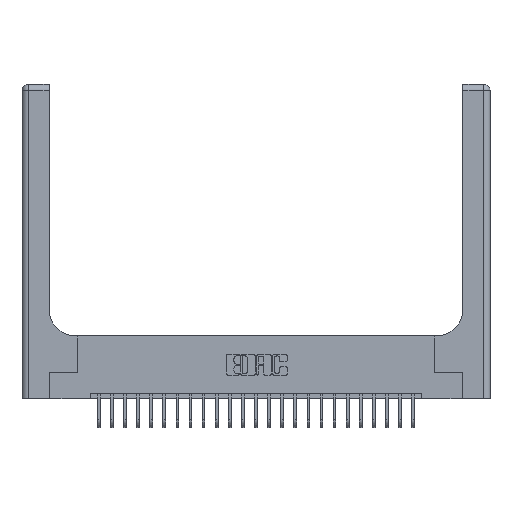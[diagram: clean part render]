
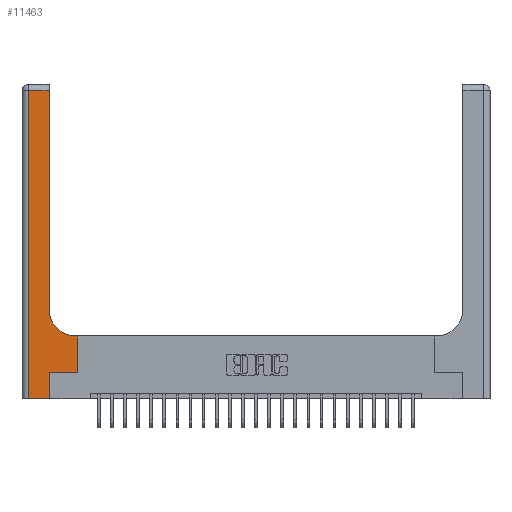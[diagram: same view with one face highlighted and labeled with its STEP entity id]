
A CAD part, top view. The second image highlights one B-rep face of the part: STEP entity #11463.
In plain terms, the highlighted planar face has unit normal (0, 0, 1).
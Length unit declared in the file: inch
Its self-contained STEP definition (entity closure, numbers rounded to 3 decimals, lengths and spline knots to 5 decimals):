
#179 = DIRECTION ( 'NONE',  ( 1., 0., 0. ) ) ;
#959 = CARTESIAN_POINT ( 'NONE',  ( 0.265, 0., 0.37 ) ) ;
#1138 = VERTEX_POINT ( 'NONE', #7204 ) ;
#1394 = LINE ( 'NONE', #23034, #22798 ) ;
#1745 = VERTEX_POINT ( 'NONE', #2069 ) ;
#1804 = ORIENTED_EDGE ( 'NONE', *, *, #21314, .T. ) ;
#2069 = CARTESIAN_POINT ( 'NONE',  ( 0.26, 2.94, 0.37 ) ) ;
#2202 = VERTEX_POINT ( 'NONE', #959 ) ;
#2420 = VECTOR ( 'NONE', #19166, 39.37008 ) ;
#2476 = DIRECTION ( 'NONE',  ( 0., 0., -1. ) ) ;
#2737 = VECTOR ( 'NONE', #9214, 39.37008 ) ;
#3122 = CIRCLE ( 'NONE', #4648, 0.25 ) ;
#3343 = AXIS2_PLACEMENT_3D ( 'NONE', #16476, #2476, #16950 ) ;
#3345 = ORIENTED_EDGE ( 'NONE', *, *, #22056, .T. ) ;
#3838 = CARTESIAN_POINT ( 'NONE',  ( 0.265, 0.25, 0.37 ) ) ;
#4006 = LINE ( 'NONE', #11257, #11906 ) ;
#4091 = LINE ( 'NONE', #20139, #2737 ) ;
#4648 = AXIS2_PLACEMENT_3D ( 'NONE', #20029, #17766, #179 ) ;
#4684 = CARTESIAN_POINT ( 'NONE',  ( 0.265, 0., 0.37 ) ) ;
#4686 = VECTOR ( 'NONE', #21534, 39.37008 ) ;
#5141 = ORIENTED_EDGE ( 'NONE', *, *, #15487, .T. ) ;
#5662 = ORIENTED_EDGE ( 'NONE', *, *, #13531, .T. ) ;
#5741 = CARTESIAN_POINT ( 'NONE',  ( 0.26, 0.6, 0.37 ) ) ;
#7204 = CARTESIAN_POINT ( 'NONE',  ( 0.26, 0.85, 0.37 ) ) ;
#7446 = ORIENTED_EDGE ( 'NONE', *, *, #13442, .T. ) ;
#8246 = VECTOR ( 'NONE', #8964, 39.37008 ) ;
#8887 = DIRECTION ( 'NONE',  ( 0., 1., 0. ) ) ;
#8964 = DIRECTION ( 'NONE',  ( -1., 0., 0. ) ) ;
#8998 = DIRECTION ( 'NONE',  ( -1., 0., 0. ) ) ;
#9214 = DIRECTION ( 'NONE',  ( 0., -1., 0. ) ) ;
#9449 = VECTOR ( 'NONE', #9553, 39.37008 ) ;
#9553 = DIRECTION ( 'NONE',  ( 1., 0., 0. ) ) ;
#9569 = EDGE_CURVE ( 'NONE', #12038, #19665, #18457, .T. ) ;
#9696 = CARTESIAN_POINT ( 'NONE',  ( 0.528, 0.25, 0.37 ) ) ;
#10384 = DIRECTION ( 'NONE',  ( 1., 0., 0. ) ) ;
#10613 = LINE ( 'NONE', #19649, #17385 ) ;
#10897 = ORIENTED_EDGE ( 'NONE', *, *, #22872, .T. ) ;
#11257 = CARTESIAN_POINT ( 'NONE',  ( 0.528, 0.25, 0.37 ) ) ;
#11463 = ADVANCED_FACE ( 'NONE', ( #18506 ), #18740, .F. ) ;
#11906 = VECTOR ( 'NONE', #8887, 39.37008 ) ;
#12038 = VERTEX_POINT ( 'NONE', #18829 ) ;
#12727 = CARTESIAN_POINT ( 'NONE',  ( 0.26, 3., 0.37 ) ) ;
#12927 = EDGE_LOOP ( 'NONE', ( #3345, #5141, #17344, #7446, #20315, #5662, #10897, #23105, #1804 ) ) ;
#13080 = VERTEX_POINT ( 'NONE', #18246 ) ;
#13442 = EDGE_CURVE ( 'NONE', #19148, #2202, #10613, .T. ) ;
#13531 = EDGE_CURVE ( 'NONE', #16179, #17462, #14645, .T. ) ;
#14645 = LINE ( 'NONE', #3838, #9449 ) ;
#15487 = EDGE_CURVE ( 'NONE', #1745, #13080, #1394, .T. ) ;
#15999 = CARTESIAN_POINT ( 'NONE',  ( 0.51, 0.6, 0.37 ) ) ;
#16179 = VERTEX_POINT ( 'NONE', #19897 ) ;
#16476 = CARTESIAN_POINT ( 'NONE',  ( 0., 3., 0.37 ) ) ;
#16950 = DIRECTION ( 'NONE',  ( -1., 0., 0. ) ) ;
#17121 = CARTESIAN_POINT ( 'NONE',  ( 0.06, 0., 0.37 ) ) ;
#17344 = ORIENTED_EDGE ( 'NONE', *, *, #17358, .T. ) ;
#17358 = EDGE_CURVE ( 'NONE', #13080, #19148, #4091, .T. ) ;
#17385 = VECTOR ( 'NONE', #10384, 39.37008 ) ;
#17462 = VERTEX_POINT ( 'NONE', #9696 ) ;
#17766 = DIRECTION ( 'NONE',  ( 0., 0., -1. ) ) ;
#18246 = CARTESIAN_POINT ( 'NONE',  ( 0.06, 2.94, 0.37 ) ) ;
#18457 = LINE ( 'NONE', #5741, #8246 ) ;
#18506 = FACE_OUTER_BOUND ( 'NONE', #12927, .T. ) ;
#18740 = PLANE ( 'NONE',  #3343 ) ;
#18829 = CARTESIAN_POINT ( 'NONE',  ( 0.528, 0.6, 0.37 ) ) ;
#18868 = EDGE_CURVE ( 'NONE', #2202, #16179, #20958, .T. ) ;
#19148 = VERTEX_POINT ( 'NONE', #17121 ) ;
#19166 = DIRECTION ( 'NONE',  ( 0., 1., 0. ) ) ;
#19649 = CARTESIAN_POINT ( 'NONE',  ( 0., 0., 0.37 ) ) ;
#19665 = VERTEX_POINT ( 'NONE', #15999 ) ;
#19897 = CARTESIAN_POINT ( 'NONE',  ( 0.265, 0.25, 0.37 ) ) ;
#20029 = CARTESIAN_POINT ( 'NONE',  ( 0.51, 0.85, 0.37 ) ) ;
#20139 = CARTESIAN_POINT ( 'NONE',  ( 0.06, 3., 0.37 ) ) ;
#20315 = ORIENTED_EDGE ( 'NONE', *, *, #18868, .T. ) ;
#20958 = LINE ( 'NONE', #4684, #2420 ) ;
#21314 = EDGE_CURVE ( 'NONE', #19665, #1138, #3122, .T. ) ;
#21411 = LINE ( 'NONE', #12727, #4686 ) ;
#21534 = DIRECTION ( 'NONE',  ( 0., 1., 0. ) ) ;
#22056 = EDGE_CURVE ( 'NONE', #1138, #1745, #21411, .T. ) ;
#22798 = VECTOR ( 'NONE', #8998, 39.37008 ) ;
#22872 = EDGE_CURVE ( 'NONE', #17462, #12038, #4006, .T. ) ;
#23034 = CARTESIAN_POINT ( 'NONE',  ( 0., 2.94, 0.37 ) ) ;
#23105 = ORIENTED_EDGE ( 'NONE', *, *, #9569, .T. ) ;
